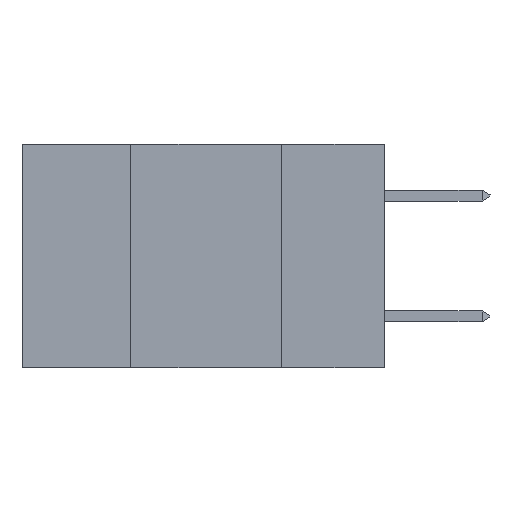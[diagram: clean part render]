
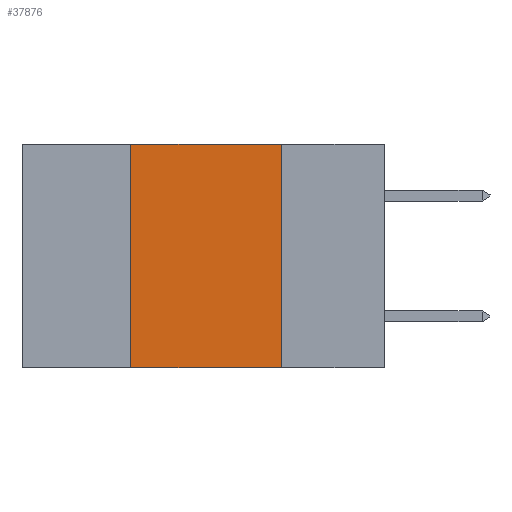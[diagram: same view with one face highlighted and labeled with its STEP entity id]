
A CAD part, left-side view. The second image highlights one B-rep face of the part: STEP entity #37876.
In plain terms, the highlighted planar face has unit normal (-1, 0, 0).
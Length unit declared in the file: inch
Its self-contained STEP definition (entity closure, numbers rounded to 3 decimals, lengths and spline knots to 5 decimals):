
#724 = PLANE ( 'NONE',  #8285 ) ;
#836 = CARTESIAN_POINT ( 'NONE',  ( 0., 0.17, 0. ) ) ;
#998 = VECTOR ( 'NONE', #30014, 39.37008 ) ;
#1854 = CARTESIAN_POINT ( 'NONE',  ( 0., 0.6, -0.37 ) ) ;
#2449 = CARTESIAN_POINT ( 'NONE',  ( 0., 0.42, 0. ) ) ;
#3549 = EDGE_CURVE ( 'NONE', #10771, #16053, #7892, .T. ) ;
#3867 = DIRECTION ( 'NONE',  ( 0., 0., -1. ) ) ;
#4313 = CARTESIAN_POINT ( 'NONE',  ( 0., 0.6, 0. ) ) ;
#4645 = ORIENTED_EDGE ( 'NONE', *, *, #16904, .F. ) ;
#4874 = VECTOR ( 'NONE', #16511, 39.37008 ) ;
#7892 = LINE ( 'NONE', #1854, #19917 ) ;
#8285 = AXIS2_PLACEMENT_3D ( 'NONE', #30133, #26847, #3867 ) ;
#9667 = LINE ( 'NONE', #836, #39823 ) ;
#10074 = CARTESIAN_POINT ( 'NONE',  ( 0., 0.17, -0.37 ) ) ;
#10738 = CARTESIAN_POINT ( 'NONE',  ( 0., 0.42, 0. ) ) ;
#10771 = VERTEX_POINT ( 'NONE', #31826 ) ;
#11857 = ORIENTED_EDGE ( 'NONE', *, *, #18274, .F. ) ;
#12276 = FACE_OUTER_BOUND ( 'NONE', #37164, .T. ) ;
#13165 = CARTESIAN_POINT ( 'NONE',  ( 0., 0.17, 0. ) ) ;
#16053 = VERTEX_POINT ( 'NONE', #10074 ) ;
#16511 = DIRECTION ( 'NONE',  ( 0., 0., 1. ) ) ;
#16904 = EDGE_CURVE ( 'NONE', #18444, #16053, #9667, .T. ) ;
#17302 = DIRECTION ( 'NONE',  ( 0., 0., -1. ) ) ;
#18126 = LINE ( 'NONE', #4313, #998 ) ;
#18274 = EDGE_CURVE ( 'NONE', #38184, #18444, #18126, .T. ) ;
#18444 = VERTEX_POINT ( 'NONE', #13165 ) ;
#19917 = VECTOR ( 'NONE', #37421, 39.37008 ) ;
#26847 = DIRECTION ( 'NONE',  ( 1., 0., 0. ) ) ;
#28361 = ORIENTED_EDGE ( 'NONE', *, *, #3549, .T. ) ;
#30014 = DIRECTION ( 'NONE',  ( 0., -1., 0. ) ) ;
#30133 = CARTESIAN_POINT ( 'NONE',  ( 0., 0.6, 0. ) ) ;
#31826 = CARTESIAN_POINT ( 'NONE',  ( 0., 0.42, -0.37 ) ) ;
#32006 = EDGE_CURVE ( 'NONE', #10771, #38184, #32508, .T. ) ;
#32338 = ORIENTED_EDGE ( 'NONE', *, *, #32006, .F. ) ;
#32508 = LINE ( 'NONE', #10738, #4874 ) ;
#37164 = EDGE_LOOP ( 'NONE', ( #4645, #11857, #32338, #28361 ) ) ;
#37421 = DIRECTION ( 'NONE',  ( 0., -1., 0. ) ) ;
#37876 = ADVANCED_FACE ( 'NONE', ( #12276 ), #724, .F. ) ;
#38184 = VERTEX_POINT ( 'NONE', #2449 ) ;
#39823 = VECTOR ( 'NONE', #17302, 39.37008 ) ;
